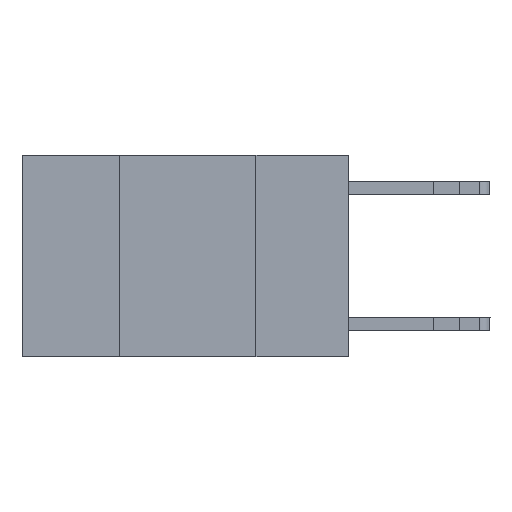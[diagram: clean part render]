
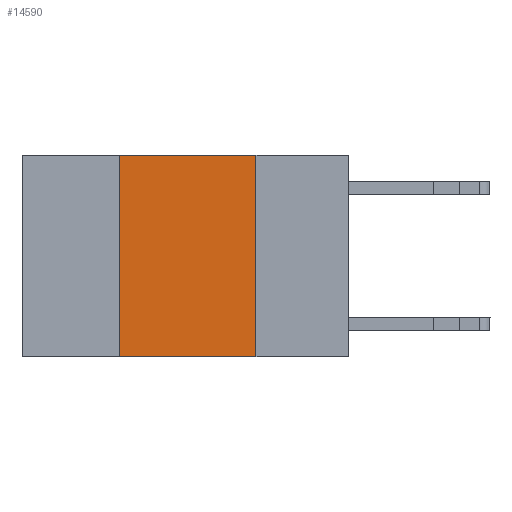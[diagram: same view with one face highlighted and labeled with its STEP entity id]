
A CAD part, left-side view. The second image highlights one B-rep face of the part: STEP entity #14590.
In plain terms, the highlighted planar face has unit normal (-1, 0, 0).
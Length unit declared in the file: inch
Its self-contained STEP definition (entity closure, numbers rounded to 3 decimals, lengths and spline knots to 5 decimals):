
#151 = EDGE_LOOP ( 'NONE', ( #18453, #19491, #19985, #20001 ) ) ;
#632 = LINE ( 'NONE', #8385, #900 ) ;
#900 = VECTOR ( 'NONE', #8305, 39.37008 ) ;
#1354 = VERTEX_POINT ( 'NONE', #24684 ) ;
#1359 = DIRECTION ( 'NONE',  ( 0., 0., 1. ) ) ;
#1939 = EDGE_CURVE ( 'NONE', #4749, #1354, #14672, .T. ) ;
#2058 = CARTESIAN_POINT ( 'NONE',  ( 0., 0.17, 0. ) ) ;
#3345 = VECTOR ( 'NONE', #19373, 39.37008 ) ;
#3886 = EDGE_CURVE ( 'NONE', #12547, #1354, #632, .T. ) ;
#4671 = EDGE_CURVE ( 'NONE', #18373, #4749, #17589, .T. ) ;
#4749 = VERTEX_POINT ( 'NONE', #2058 ) ;
#6551 = EDGE_CURVE ( 'NONE', #12547, #18373, #9951, .T. ) ;
#8305 = DIRECTION ( 'NONE',  ( 0., -1., 0. ) ) ;
#8385 = CARTESIAN_POINT ( 'NONE',  ( 0., 0.6, -0.37 ) ) ;
#9328 = VECTOR ( 'NONE', #1359, 39.37008 ) ;
#9951 = LINE ( 'NONE', #15103, #9328 ) ;
#11962 = DIRECTION ( 'NONE',  ( 0., 0., -1. ) ) ;
#12333 = DIRECTION ( 'NONE',  ( 0., 0., -1. ) ) ;
#12433 = CARTESIAN_POINT ( 'NONE',  ( 0., 0.17, 0. ) ) ;
#12547 = VERTEX_POINT ( 'NONE', #23329 ) ;
#14484 = VECTOR ( 'NONE', #11962, 39.37008 ) ;
#14590 = ADVANCED_FACE ( 'NONE', ( #23152 ), #19937, .F. ) ;
#14672 = LINE ( 'NONE', #12433, #14484 ) ;
#15103 = CARTESIAN_POINT ( 'NONE',  ( 0., 0.42, 0. ) ) ;
#16790 = AXIS2_PLACEMENT_3D ( 'NONE', #21848, #23794, #12333 ) ;
#17589 = LINE ( 'NONE', #24995, #3345 ) ;
#18373 = VERTEX_POINT ( 'NONE', #19155 ) ;
#18453 = ORIENTED_EDGE ( 'NONE', *, *, #1939, .F. ) ;
#19155 = CARTESIAN_POINT ( 'NONE',  ( 0., 0.42, 0. ) ) ;
#19373 = DIRECTION ( 'NONE',  ( 0., -1., 0. ) ) ;
#19491 = ORIENTED_EDGE ( 'NONE', *, *, #4671, .F. ) ;
#19937 = PLANE ( 'NONE',  #16790 ) ;
#19985 = ORIENTED_EDGE ( 'NONE', *, *, #6551, .F. ) ;
#20001 = ORIENTED_EDGE ( 'NONE', *, *, #3886, .T. ) ;
#21848 = CARTESIAN_POINT ( 'NONE',  ( 0., 0.6, 0. ) ) ;
#23152 = FACE_OUTER_BOUND ( 'NONE', #151, .T. ) ;
#23329 = CARTESIAN_POINT ( 'NONE',  ( 0., 0.42, -0.37 ) ) ;
#23794 = DIRECTION ( 'NONE',  ( 1., 0., 0. ) ) ;
#24684 = CARTESIAN_POINT ( 'NONE',  ( 0., 0.17, -0.37 ) ) ;
#24995 = CARTESIAN_POINT ( 'NONE',  ( 0., 0.6, 0. ) ) ;
